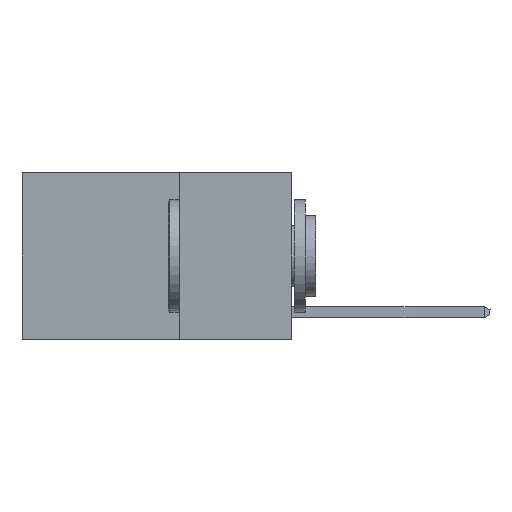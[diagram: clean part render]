
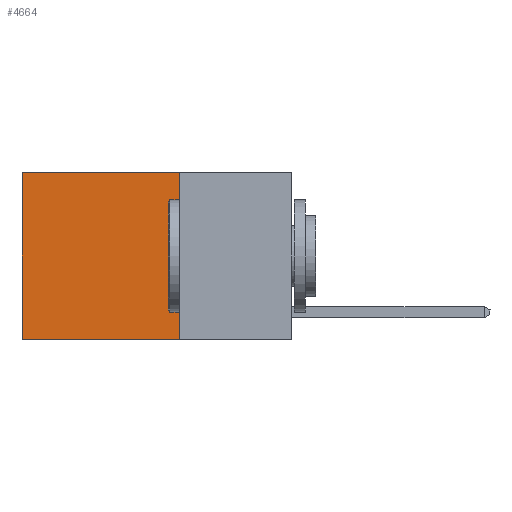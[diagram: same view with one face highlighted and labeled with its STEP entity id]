
A CAD part, left-side view. The second image highlights one B-rep face of the part: STEP entity #4664.
In plain terms, the highlighted planar face has unit normal (-1, 0, 0).
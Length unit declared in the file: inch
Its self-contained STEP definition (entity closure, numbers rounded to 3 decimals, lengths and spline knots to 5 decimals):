
#629 = EDGE_CURVE ( 'NONE', #2962, #8115, #6306, .T. ) ;
#2220 = CARTESIAN_POINT ( 'NONE',  ( 0.2625, 0.25, 0. ) ) ;
#2849 = ORIENTED_EDGE ( 'NONE', *, *, #4925, .F. ) ;
#2962 = VERTEX_POINT ( 'NONE', #12358 ) ;
#3316 = ORIENTED_EDGE ( 'NONE', *, *, #10372, .T. ) ;
#4488 = EDGE_LOOP ( 'NONE', ( #11958, #12924, #2849, #3316 ) ) ;
#4664 = ADVANCED_FACE ( 'NONE', ( #5982 ), #9325, .F. ) ;
#4925 = EDGE_CURVE ( 'NONE', #14902, #12402, #9211, .T. ) ;
#5228 = CARTESIAN_POINT ( 'NONE',  ( 0.2625, 0.6, -0.37 ) ) ;
#5555 = CARTESIAN_POINT ( 'NONE',  ( 0.2625, 0.25, -0.37 ) ) ;
#5567 = VECTOR ( 'NONE', #7150, 39.37008 ) ;
#5928 = AXIS2_PLACEMENT_3D ( 'NONE', #14334, #6796, #15541 ) ;
#5980 = DIRECTION ( 'NONE',  ( 0., 0., -1. ) ) ;
#5982 = FACE_OUTER_BOUND ( 'NONE', #4488, .T. ) ;
#6306 = LINE ( 'NONE', #10150, #15526 ) ;
#6796 = DIRECTION ( 'NONE',  ( 1., 0., 0. ) ) ;
#6862 = DIRECTION ( 'NONE',  ( 0., 1., 0. ) ) ;
#7150 = DIRECTION ( 'NONE',  ( 0., 1., 0. ) ) ;
#8094 = CARTESIAN_POINT ( 'NONE',  ( 0.2625, 0.25, -0.37 ) ) ;
#8115 = VERTEX_POINT ( 'NONE', #5228 ) ;
#8582 = DIRECTION ( 'NONE',  ( 0., 0., -1. ) ) ;
#9211 = LINE ( 'NONE', #12304, #15411 ) ;
#9325 = PLANE ( 'NONE',  #5928 ) ;
#10150 = CARTESIAN_POINT ( 'NONE',  ( 0.2625, 0.6, 0. ) ) ;
#10231 = EDGE_CURVE ( 'NONE', #12402, #8115, #14278, .T. ) ;
#10372 = EDGE_CURVE ( 'NONE', #14902, #2962, #12371, .T. ) ;
#11013 = VECTOR ( 'NONE', #6862, 39.37008 ) ;
#11958 = ORIENTED_EDGE ( 'NONE', *, *, #629, .T. ) ;
#12304 = CARTESIAN_POINT ( 'NONE',  ( 0.2625, 0.25, 0. ) ) ;
#12358 = CARTESIAN_POINT ( 'NONE',  ( 0.2625, 0.6, 0. ) ) ;
#12371 = LINE ( 'NONE', #15874, #5567 ) ;
#12402 = VERTEX_POINT ( 'NONE', #8094 ) ;
#12924 = ORIENTED_EDGE ( 'NONE', *, *, #10231, .F. ) ;
#14278 = LINE ( 'NONE', #5555, #11013 ) ;
#14334 = CARTESIAN_POINT ( 'NONE',  ( 0.2625, 0.25, 0. ) ) ;
#14902 = VERTEX_POINT ( 'NONE', #2220 ) ;
#15411 = VECTOR ( 'NONE', #5980, 39.37008 ) ;
#15526 = VECTOR ( 'NONE', #8582, 39.37008 ) ;
#15541 = DIRECTION ( 'NONE',  ( 0., 0., -1. ) ) ;
#15874 = CARTESIAN_POINT ( 'NONE',  ( 0.2625, 0.25, 0. ) ) ;
